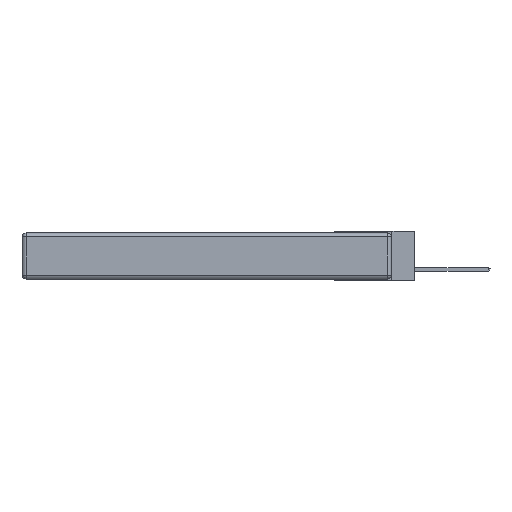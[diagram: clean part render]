
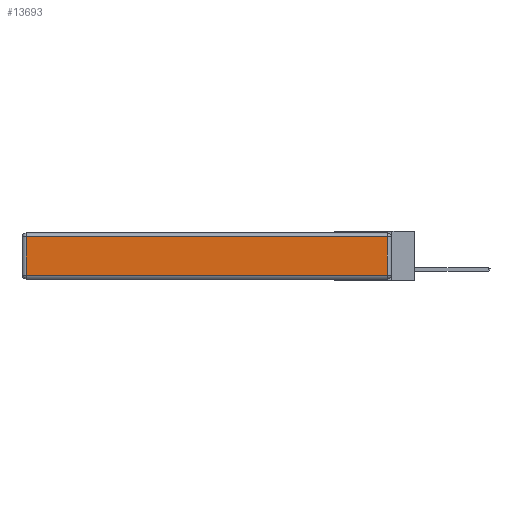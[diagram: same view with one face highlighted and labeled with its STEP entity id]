
A CAD part, left-side view. The second image highlights one B-rep face of the part: STEP entity #13693.
In plain terms, the highlighted planar face has unit normal (-1, 0, 0).
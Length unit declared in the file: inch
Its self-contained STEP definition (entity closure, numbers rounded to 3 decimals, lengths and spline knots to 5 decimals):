
#1682 = CARTESIAN_POINT ( 'NONE',  ( 0., 2.72, -0.343 ) ) ;
#2093 = ORIENTED_EDGE ( 'NONE', *, *, #9583, .T. ) ;
#2107 = DIRECTION ( 'NONE',  ( 0., 0., 1. ) ) ;
#2313 = EDGE_LOOP ( 'NONE', ( #14911, #13571, #2093, #10204 ) ) ;
#2808 = LINE ( 'NONE', #9489, #10472 ) ;
#3055 = CARTESIAN_POINT ( 'NONE',  ( 0., 0.03, -0.313 ) ) ;
#3118 = EDGE_CURVE ( 'NONE', #3861, #8191, #2808, .T. ) ;
#3417 = PLANE ( 'NONE',  #4375 ) ;
#3861 = VERTEX_POINT ( 'NONE', #3055 ) ;
#3863 = EDGE_CURVE ( 'NONE', #5252, #4430, #12443, .T. ) ;
#4375 = AXIS2_PLACEMENT_3D ( 'NONE', #11563, #13758, #2107 ) ;
#4430 = VERTEX_POINT ( 'NONE', #14940 ) ;
#4494 = LINE ( 'NONE', #6676, #8694 ) ;
#5252 = VERTEX_POINT ( 'NONE', #14340 ) ;
#6676 = CARTESIAN_POINT ( 'NONE',  ( 0., 0., -0.313 ) ) ;
#7003 = DIRECTION ( 'NONE',  ( 0., 0., 1. ) ) ;
#7955 = LINE ( 'NONE', #12432, #9792 ) ;
#7968 = FACE_OUTER_BOUND ( 'NONE', #2313, .T. ) ;
#8065 = VECTOR ( 'NONE', #12213, 39.37008 ) ;
#8191 = VERTEX_POINT ( 'NONE', #12513 ) ;
#8694 = VECTOR ( 'NONE', #9121, 39.37008 ) ;
#9121 = DIRECTION ( 'NONE',  ( 0., -1., 0. ) ) ;
#9286 = EDGE_CURVE ( 'NONE', #4430, #3861, #4494, .T. ) ;
#9489 = CARTESIAN_POINT ( 'NONE',  ( 0., 0.03, -0.343 ) ) ;
#9583 = EDGE_CURVE ( 'NONE', #8191, #5252, #7955, .T. ) ;
#9792 = VECTOR ( 'NONE', #12208, 39.37008 ) ;
#10204 = ORIENTED_EDGE ( 'NONE', *, *, #3863, .T. ) ;
#10472 = VECTOR ( 'NONE', #7003, 39.37008 ) ;
#11563 = CARTESIAN_POINT ( 'NONE',  ( 0., 0., -0.343 ) ) ;
#12208 = DIRECTION ( 'NONE',  ( 0., 1., 0. ) ) ;
#12213 = DIRECTION ( 'NONE',  ( 0., 0., -1. ) ) ;
#12432 = CARTESIAN_POINT ( 'NONE',  ( 0., 2.75, -0.03 ) ) ;
#12443 = LINE ( 'NONE', #1682, #8065 ) ;
#12513 = CARTESIAN_POINT ( 'NONE',  ( 0., 0.03, -0.03 ) ) ;
#13571 = ORIENTED_EDGE ( 'NONE', *, *, #3118, .T. ) ;
#13693 = ADVANCED_FACE ( 'NONE', ( #7968 ), #3417, .T. ) ;
#13758 = DIRECTION ( 'NONE',  ( -1., 0., 0. ) ) ;
#14340 = CARTESIAN_POINT ( 'NONE',  ( 0., 2.72, -0.03 ) ) ;
#14911 = ORIENTED_EDGE ( 'NONE', *, *, #9286, .T. ) ;
#14940 = CARTESIAN_POINT ( 'NONE',  ( 0., 2.72, -0.313 ) ) ;
